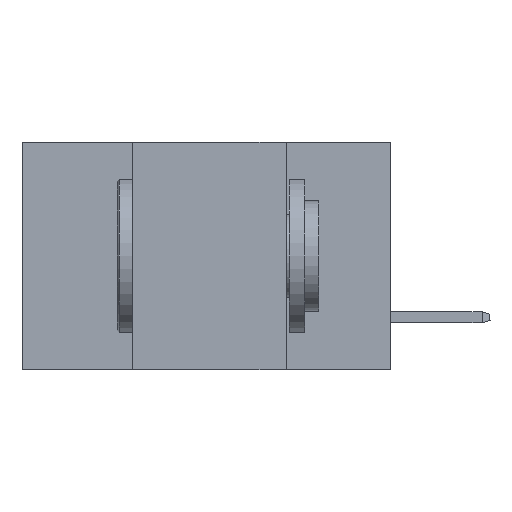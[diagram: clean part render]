
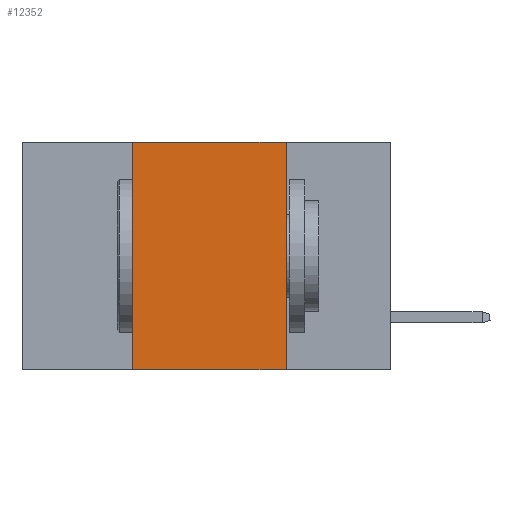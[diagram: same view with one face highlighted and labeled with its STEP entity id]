
A CAD part, left-side view. The second image highlights one B-rep face of the part: STEP entity #12352.
In plain terms, the highlighted planar face has unit normal (-1, 0, 0).
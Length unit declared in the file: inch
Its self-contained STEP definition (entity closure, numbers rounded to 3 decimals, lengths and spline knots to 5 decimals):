
#20 = VECTOR ( 'NONE', #4458, 39.37008 ) ;
#81 = CARTESIAN_POINT ( 'NONE',  ( 0., 0.17, 0. ) ) ;
#344 = CARTESIAN_POINT ( 'NONE',  ( 0., 0.42, 0. ) ) ;
#630 = EDGE_CURVE ( 'NONE', #5130, #5425, #13158, .T. ) ;
#749 = ORIENTED_EDGE ( 'NONE', *, *, #836, .F. ) ;
#781 = ORIENTED_EDGE ( 'NONE', *, *, #12601, .F. ) ;
#836 = EDGE_CURVE ( 'NONE', #8885, #5425, #5793, .T. ) ;
#1152 = DIRECTION ( 'NONE',  ( 0., 0., -1. ) ) ;
#1627 = CARTESIAN_POINT ( 'NONE',  ( 0., 0.17, -0.37 ) ) ;
#1704 = VERTEX_POINT ( 'NONE', #12156 ) ;
#2283 = EDGE_CURVE ( 'NONE', #1704, #8885, #7433, .T. ) ;
#2340 = PLANE ( 'NONE',  #3824 ) ;
#2515 = ORIENTED_EDGE ( 'NONE', *, *, #2283, .F. ) ;
#3824 = AXIS2_PLACEMENT_3D ( 'NONE', #6712, #5684, #1152 ) ;
#4458 = DIRECTION ( 'NONE',  ( 0., 0., -1. ) ) ;
#5130 = VERTEX_POINT ( 'NONE', #5387 ) ;
#5387 = CARTESIAN_POINT ( 'NONE',  ( 0., 0.42, -0.37 ) ) ;
#5425 = VERTEX_POINT ( 'NONE', #1627 ) ;
#5684 = DIRECTION ( 'NONE',  ( 1., 0., 0. ) ) ;
#5793 = LINE ( 'NONE', #81, #20 ) ;
#6500 = CARTESIAN_POINT ( 'NONE',  ( 0., 0.6, -0.37 ) ) ;
#6712 = CARTESIAN_POINT ( 'NONE',  ( 0., 0.6, 0. ) ) ;
#6813 = EDGE_LOOP ( 'NONE', ( #749, #2515, #781, #8912 ) ) ;
#7433 = LINE ( 'NONE', #12499, #10753 ) ;
#7566 = DIRECTION ( 'NONE',  ( 0., -1., 0. ) ) ;
#7732 = CARTESIAN_POINT ( 'NONE',  ( 0., 0.17, 0. ) ) ;
#8319 = DIRECTION ( 'NONE',  ( 0., 0., 1. ) ) ;
#8885 = VERTEX_POINT ( 'NONE', #7732 ) ;
#8912 = ORIENTED_EDGE ( 'NONE', *, *, #630, .T. ) ;
#10155 = VECTOR ( 'NONE', #7566, 39.37008 ) ;
#10753 = VECTOR ( 'NONE', #11147, 39.37008 ) ;
#11147 = DIRECTION ( 'NONE',  ( 0., -1., 0. ) ) ;
#12130 = FACE_OUTER_BOUND ( 'NONE', #6813, .T. ) ;
#12156 = CARTESIAN_POINT ( 'NONE',  ( 0., 0.42, 0. ) ) ;
#12352 = ADVANCED_FACE ( 'NONE', ( #12130 ), #2340, .F. ) ;
#12499 = CARTESIAN_POINT ( 'NONE',  ( 0., 0.6, 0. ) ) ;
#12601 = EDGE_CURVE ( 'NONE', #5130, #1704, #13572, .T. ) ;
#13158 = LINE ( 'NONE', #6500, #10155 ) ;
#13572 = LINE ( 'NONE', #344, #13741 ) ;
#13741 = VECTOR ( 'NONE', #8319, 39.37008 ) ;
